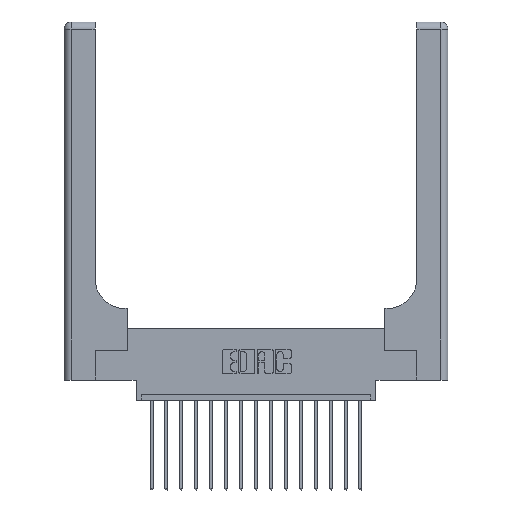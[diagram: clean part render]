
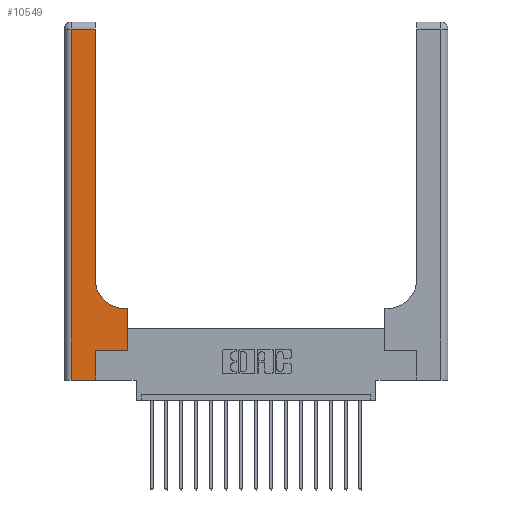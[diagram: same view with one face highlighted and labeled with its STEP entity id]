
A CAD part, top view. The second image highlights one B-rep face of the part: STEP entity #10549.
In plain terms, the highlighted planar face has unit normal (0, 0, 1).
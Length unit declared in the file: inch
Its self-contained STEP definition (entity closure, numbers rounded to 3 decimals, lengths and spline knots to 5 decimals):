
#198 = DIRECTION ( 'NONE',  ( 0., 0., -1. ) ) ;
#768 = LINE ( 'NONE', #6175, #7592 ) ;
#1597 = CARTESIAN_POINT ( 'NONE',  ( 0., 2.94, 0.37 ) ) ;
#1769 = LINE ( 'NONE', #4123, #1974 ) ;
#1876 = VECTOR ( 'NONE', #6711, 39.37008 ) ;
#1974 = VECTOR ( 'NONE', #16685, 39.37008 ) ;
#2162 = CARTESIAN_POINT ( 'NONE',  ( 0.265, 0.25, 0.37 ) ) ;
#2981 = EDGE_CURVE ( 'NONE', #17175, #18172, #14340, .T. ) ;
#3082 = DIRECTION ( 'NONE',  ( 1., 0., 0. ) ) ;
#3127 = ORIENTED_EDGE ( 'NONE', *, *, #3407, .T. ) ;
#3198 = EDGE_CURVE ( 'NONE', #14525, #17175, #8102, .T. ) ;
#3407 = EDGE_CURVE ( 'NONE', #9714, #8745, #5935, .T. ) ;
#3866 = VECTOR ( 'NONE', #5037, 39.37008 ) ;
#4123 = CARTESIAN_POINT ( 'NONE',  ( 0.26, 0.6, 0.37 ) ) ;
#4315 = CARTESIAN_POINT ( 'NONE',  ( 0.528, 0.25, 0.37 ) ) ;
#4791 = EDGE_CURVE ( 'NONE', #10776, #9714, #17772, .T. ) ;
#5037 = DIRECTION ( 'NONE',  ( 1., 0., 0. ) ) ;
#5531 = VECTOR ( 'NONE', #16967, 39.37008 ) ;
#5578 = CARTESIAN_POINT ( 'NONE',  ( 0.06, 0., 0.37 ) ) ;
#5935 = LINE ( 'NONE', #11804, #8750 ) ;
#6122 = CARTESIAN_POINT ( 'NONE',  ( 0., 0., 0.37 ) ) ;
#6175 = CARTESIAN_POINT ( 'NONE',  ( 0.265, 0., 0.37 ) ) ;
#6711 = DIRECTION ( 'NONE',  ( 0., 1., 0. ) ) ;
#6926 = VERTEX_POINT ( 'NONE', #8376 ) ;
#7066 = DIRECTION ( 'NONE',  ( 1., 0., 0. ) ) ;
#7272 = ORIENTED_EDGE ( 'NONE', *, *, #3198, .T. ) ;
#7392 = EDGE_CURVE ( 'NONE', #18172, #13918, #11111, .T. ) ;
#7592 = VECTOR ( 'NONE', #11717, 39.37008 ) ;
#7602 = DIRECTION ( 'NONE',  ( 0., 1., 0. ) ) ;
#7752 = CARTESIAN_POINT ( 'NONE',  ( 0., 3., 0.37 ) ) ;
#8102 = LINE ( 'NONE', #1597, #14322 ) ;
#8376 = CARTESIAN_POINT ( 'NONE',  ( 0.51, 0.6, 0.37 ) ) ;
#8745 = VERTEX_POINT ( 'NONE', #9256 ) ;
#8750 = VECTOR ( 'NONE', #7602, 39.37008 ) ;
#9138 = EDGE_CURVE ( 'NONE', #13918, #10776, #768, .T. ) ;
#9256 = CARTESIAN_POINT ( 'NONE',  ( 0.528, 0.6, 0.37 ) ) ;
#9307 = EDGE_CURVE ( 'NONE', #17242, #14525, #12689, .T. ) ;
#9714 = VERTEX_POINT ( 'NONE', #4315 ) ;
#9724 = ORIENTED_EDGE ( 'NONE', *, *, #9307, .T. ) ;
#10312 = CARTESIAN_POINT ( 'NONE',  ( 0.26, 2.94, 0.37 ) ) ;
#10549 = ADVANCED_FACE ( 'NONE', ( #12460 ), #14879, .F. ) ;
#10642 = CARTESIAN_POINT ( 'NONE',  ( 0.26, 0.85, 0.37 ) ) ;
#10725 = VECTOR ( 'NONE', #7066, 39.37008 ) ;
#10776 = VERTEX_POINT ( 'NONE', #2162 ) ;
#10911 = CARTESIAN_POINT ( 'NONE',  ( 0.26, 3., 0.37 ) ) ;
#11111 = LINE ( 'NONE', #6122, #3866 ) ;
#11179 = AXIS2_PLACEMENT_3D ( 'NONE', #15727, #198, #3082 ) ;
#11717 = DIRECTION ( 'NONE',  ( 0., 1., 0. ) ) ;
#11804 = CARTESIAN_POINT ( 'NONE',  ( 0.528, 0.25, 0.37 ) ) ;
#12159 = DIRECTION ( 'NONE',  ( 0., 0., -1. ) ) ;
#12180 = ORIENTED_EDGE ( 'NONE', *, *, #2981, .T. ) ;
#12460 = FACE_OUTER_BOUND ( 'NONE', #15758, .T. ) ;
#12689 = LINE ( 'NONE', #10911, #1876 ) ;
#12738 = EDGE_CURVE ( 'NONE', #8745, #6926, #1769, .T. ) ;
#12882 = CIRCLE ( 'NONE', #11179, 0.25 ) ;
#13349 = DIRECTION ( 'NONE',  ( -1., 0., 0. ) ) ;
#13918 = VERTEX_POINT ( 'NONE', #14017 ) ;
#14017 = CARTESIAN_POINT ( 'NONE',  ( 0.265, 0., 0.37 ) ) ;
#14187 = CARTESIAN_POINT ( 'NONE',  ( 0.06, 3., 0.37 ) ) ;
#14318 = ORIENTED_EDGE ( 'NONE', *, *, #16937, .T. ) ;
#14322 = VECTOR ( 'NONE', #16776, 39.37008 ) ;
#14340 = LINE ( 'NONE', #14187, #5531 ) ;
#14525 = VERTEX_POINT ( 'NONE', #10312 ) ;
#14716 = CARTESIAN_POINT ( 'NONE',  ( 0.06, 2.94, 0.37 ) ) ;
#14879 = PLANE ( 'NONE',  #16119 ) ;
#15558 = ORIENTED_EDGE ( 'NONE', *, *, #12738, .T. ) ;
#15727 = CARTESIAN_POINT ( 'NONE',  ( 0.51, 0.85, 0.37 ) ) ;
#15758 = EDGE_LOOP ( 'NONE', ( #9724, #7272, #12180, #15816, #17347, #16809, #3127, #15558, #14318 ) ) ;
#15816 = ORIENTED_EDGE ( 'NONE', *, *, #7392, .T. ) ;
#16119 = AXIS2_PLACEMENT_3D ( 'NONE', #7752, #12159, #13349 ) ;
#16685 = DIRECTION ( 'NONE',  ( -1., 0., 0. ) ) ;
#16776 = DIRECTION ( 'NONE',  ( -1., 0., 0. ) ) ;
#16809 = ORIENTED_EDGE ( 'NONE', *, *, #4791, .T. ) ;
#16937 = EDGE_CURVE ( 'NONE', #6926, #17242, #12882, .T. ) ;
#16967 = DIRECTION ( 'NONE',  ( 0., -1., 0. ) ) ;
#16975 = CARTESIAN_POINT ( 'NONE',  ( 0.265, 0.25, 0.37 ) ) ;
#17175 = VERTEX_POINT ( 'NONE', #14716 ) ;
#17242 = VERTEX_POINT ( 'NONE', #10642 ) ;
#17347 = ORIENTED_EDGE ( 'NONE', *, *, #9138, .T. ) ;
#17772 = LINE ( 'NONE', #16975, #10725 ) ;
#18172 = VERTEX_POINT ( 'NONE', #5578 ) ;
